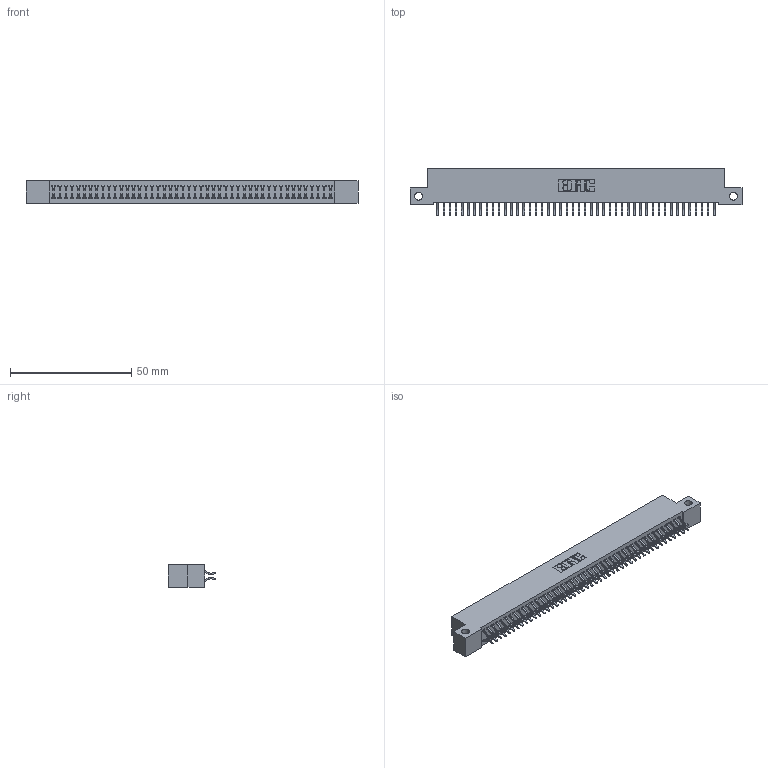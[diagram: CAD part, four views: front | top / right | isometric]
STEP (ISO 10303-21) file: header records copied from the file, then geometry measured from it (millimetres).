
FILE_DESCRIPTION (( 'STEP AP203' ), '1' );
FILE_NAME ('392-092-556-212.STEP', '2018-08-18T08:18:16', ( '' ), ( '' ), 'SwSTEP 2.0', 'SolidWorks 2016', '' );
FILE_SCHEMA (( 'CONFIG_CONTROL_DESIGN' ));
Length unit declared in the file: inch
Products named in the file (3): 342 Part_Side Mount; 345-292-001_556 Tail; 392-092-556-212
Assembly tree (93 placements, depth 2):
  392-092-556-212
    342 Part_Side Mount
    345-292-001_556 Tail  x92
Bounding box: 137.16 x 19.58 x 9.4 mm (x, y, z)
Volume: 12266.5 mm3; surface area: 19816.3 mm2
Topology: 93 solids, 93 shells, 5446 faces, 16215 edges, 10686 vertices
Faces by surface type: plane 3746, cylinder 1700
Entity records: 29167 total; most frequent: CARTESIAN_POINT 4842, ORIENTED_EDGE 4766, DIRECTION 4119, EDGE_CURVE 2383, LINE 2247, VECTOR 2247, VERTEX_POINT 1586, AXIS2_PLACEMENT_3D 936
